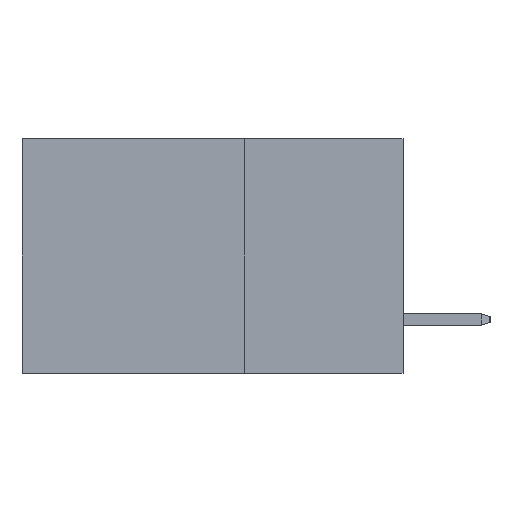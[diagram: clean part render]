
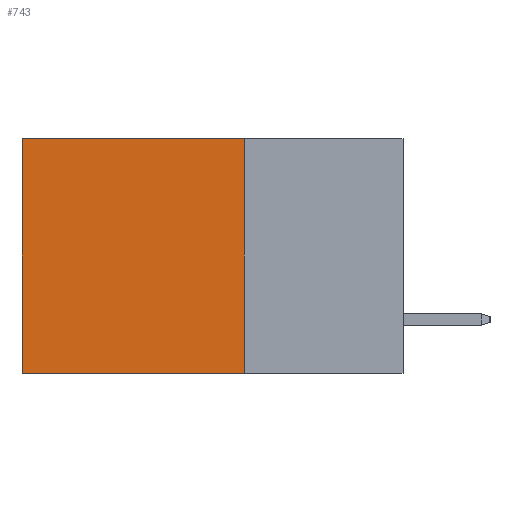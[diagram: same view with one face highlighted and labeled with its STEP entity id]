
A CAD part, left-side view. The second image highlights one B-rep face of the part: STEP entity #743.
In plain terms, the highlighted planar face has unit normal (-1, 0, 0).
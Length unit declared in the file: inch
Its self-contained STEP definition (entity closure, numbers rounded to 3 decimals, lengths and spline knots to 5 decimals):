
#81 = DIRECTION ( 'NONE',  ( 1., 0., 0. ) ) ;
#625 = VERTEX_POINT ( 'NONE', #1703 ) ;
#680 = CARTESIAN_POINT ( 'NONE',  ( 0.2875, 0.25, -0.37 ) ) ;
#743 = ADVANCED_FACE ( 'NONE', ( #2555 ), #1002, .F. ) ;
#801 = LINE ( 'NONE', #2631, #8959 ) ;
#811 = CARTESIAN_POINT ( 'NONE',  ( 0.2875, 0.6, -0.37 ) ) ;
#1002 = PLANE ( 'NONE',  #5697 ) ;
#1386 = ORIENTED_EDGE ( 'NONE', *, *, #5239, .F. ) ;
#1561 = LINE ( 'NONE', #8448, #9047 ) ;
#1703 = CARTESIAN_POINT ( 'NONE',  ( 0.2875, 0.25, 0. ) ) ;
#2373 = VECTOR ( 'NONE', #3191, 39.37008 ) ;
#2555 = FACE_OUTER_BOUND ( 'NONE', #5990, .T. ) ;
#2631 = CARTESIAN_POINT ( 'NONE',  ( 0.2875, 0.6, 0. ) ) ;
#3041 = DIRECTION ( 'NONE',  ( 0., 0., -1. ) ) ;
#3191 = DIRECTION ( 'NONE',  ( 0., 1., 0. ) ) ;
#3194 = VERTEX_POINT ( 'NONE', #8349 ) ;
#3736 = VERTEX_POINT ( 'NONE', #811 ) ;
#4161 = CARTESIAN_POINT ( 'NONE',  ( 0.2875, 0.25, -0.37 ) ) ;
#4444 = DIRECTION ( 'NONE',  ( 0., 0., -1. ) ) ;
#4477 = EDGE_CURVE ( 'NONE', #5863, #3736, #9262, .T. ) ;
#4631 = CARTESIAN_POINT ( 'NONE',  ( 0.2875, 0.25, 0. ) ) ;
#5239 = EDGE_CURVE ( 'NONE', #625, #5863, #10814, .T. ) ;
#5697 = AXIS2_PLACEMENT_3D ( 'NONE', #6021, #81, #10558 ) ;
#5863 = VERTEX_POINT ( 'NONE', #680 ) ;
#5990 = EDGE_LOOP ( 'NONE', ( #9535, #7647, #1386, #11169 ) ) ;
#6021 = CARTESIAN_POINT ( 'NONE',  ( 0.2875, 0.25, 0. ) ) ;
#6535 = VECTOR ( 'NONE', #3041, 39.37008 ) ;
#6770 = EDGE_CURVE ( 'NONE', #3194, #3736, #801, .T. ) ;
#6841 = DIRECTION ( 'NONE',  ( 0., 1., 0. ) ) ;
#7647 = ORIENTED_EDGE ( 'NONE', *, *, #4477, .F. ) ;
#8349 = CARTESIAN_POINT ( 'NONE',  ( 0.2875, 0.6, 0. ) ) ;
#8448 = CARTESIAN_POINT ( 'NONE',  ( 0.2875, 0.25, 0. ) ) ;
#8959 = VECTOR ( 'NONE', #4444, 39.37008 ) ;
#9047 = VECTOR ( 'NONE', #6841, 39.37008 ) ;
#9262 = LINE ( 'NONE', #4161, #2373 ) ;
#9535 = ORIENTED_EDGE ( 'NONE', *, *, #6770, .T. ) ;
#10221 = EDGE_CURVE ( 'NONE', #625, #3194, #1561, .T. ) ;
#10558 = DIRECTION ( 'NONE',  ( 0., 0., -1. ) ) ;
#10814 = LINE ( 'NONE', #4631, #6535 ) ;
#11169 = ORIENTED_EDGE ( 'NONE', *, *, #10221, .T. ) ;
